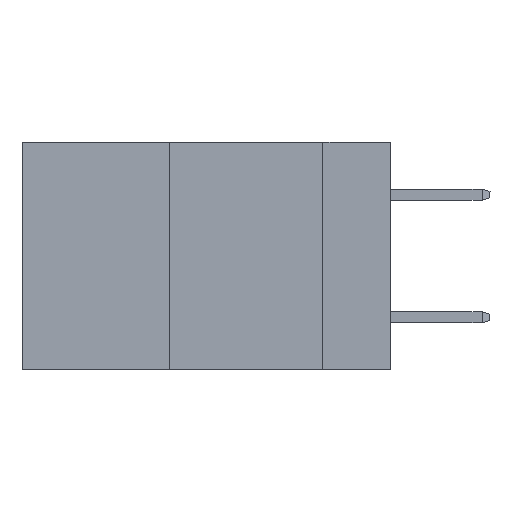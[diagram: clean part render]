
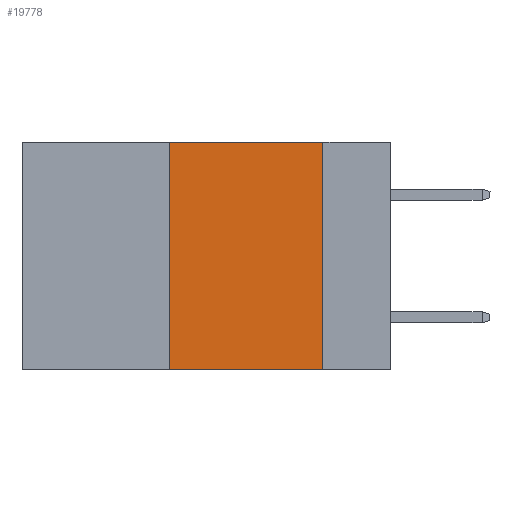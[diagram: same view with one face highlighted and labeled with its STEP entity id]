
A CAD part, left-side view. The second image highlights one B-rep face of the part: STEP entity #19778.
In plain terms, the highlighted planar face has unit normal (-1, 0, 0).
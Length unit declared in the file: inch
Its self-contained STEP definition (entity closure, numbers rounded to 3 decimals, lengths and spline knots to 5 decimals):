
#240 = DIRECTION ( 'NONE',  ( 0., 0., 1. ) ) ;
#865 = AXIS2_PLACEMENT_3D ( 'NONE', #5860, #7528, #19065 ) ;
#1571 = FACE_OUTER_BOUND ( 'NONE', #2227, .T. ) ;
#1579 = CARTESIAN_POINT ( 'NONE',  ( 0., 0.11, 0. ) ) ;
#2086 = ORIENTED_EDGE ( 'NONE', *, *, #17200, .F. ) ;
#2227 = EDGE_LOOP ( 'NONE', ( #17621, #2086, #16834, #9053 ) ) ;
#2292 = CARTESIAN_POINT ( 'NONE',  ( 0., 0.6, 0. ) ) ;
#3616 = LINE ( 'NONE', #15989, #20672 ) ;
#3717 = VECTOR ( 'NONE', #240, 39.37008 ) ;
#4188 = PLANE ( 'NONE',  #865 ) ;
#4448 = LINE ( 'NONE', #1579, #19172 ) ;
#4808 = DIRECTION ( 'NONE',  ( 0., 0., -1. ) ) ;
#4874 = EDGE_CURVE ( 'NONE', #15986, #5708, #8116, .T. ) ;
#5708 = VERTEX_POINT ( 'NONE', #14216 ) ;
#5860 = CARTESIAN_POINT ( 'NONE',  ( 0., 0.6, 0. ) ) ;
#5955 = EDGE_CURVE ( 'NONE', #6015, #7404, #4448, .T. ) ;
#6015 = VERTEX_POINT ( 'NONE', #19885 ) ;
#7088 = EDGE_CURVE ( 'NONE', #15986, #7404, #3616, .T. ) ;
#7404 = VERTEX_POINT ( 'NONE', #11786 ) ;
#7528 = DIRECTION ( 'NONE',  ( 1., 0., 0. ) ) ;
#8116 = LINE ( 'NONE', #15063, #3717 ) ;
#8850 = DIRECTION ( 'NONE',  ( 0., -1., 0. ) ) ;
#9053 = ORIENTED_EDGE ( 'NONE', *, *, #7088, .T. ) ;
#11786 = CARTESIAN_POINT ( 'NONE',  ( 0., 0.11, -0.37 ) ) ;
#12749 = CARTESIAN_POINT ( 'NONE',  ( 0., 0.36, -0.37 ) ) ;
#14216 = CARTESIAN_POINT ( 'NONE',  ( 0., 0.36, 0. ) ) ;
#15063 = CARTESIAN_POINT ( 'NONE',  ( 0., 0.36, 0. ) ) ;
#15918 = DIRECTION ( 'NONE',  ( 0., -1., 0. ) ) ;
#15986 = VERTEX_POINT ( 'NONE', #12749 ) ;
#15989 = CARTESIAN_POINT ( 'NONE',  ( 0., 0.6, -0.37 ) ) ;
#16834 = ORIENTED_EDGE ( 'NONE', *, *, #4874, .F. ) ;
#17200 = EDGE_CURVE ( 'NONE', #5708, #6015, #20229, .T. ) ;
#17621 = ORIENTED_EDGE ( 'NONE', *, *, #5955, .F. ) ;
#19065 = DIRECTION ( 'NONE',  ( 0., 0., -1. ) ) ;
#19172 = VECTOR ( 'NONE', #4808, 39.37008 ) ;
#19778 = ADVANCED_FACE ( 'NONE', ( #1571 ), #4188, .F. ) ;
#19885 = CARTESIAN_POINT ( 'NONE',  ( 0., 0.11, 0. ) ) ;
#20229 = LINE ( 'NONE', #2292, #20736 ) ;
#20672 = VECTOR ( 'NONE', #15918, 39.37008 ) ;
#20736 = VECTOR ( 'NONE', #8850, 39.37008 ) ;
